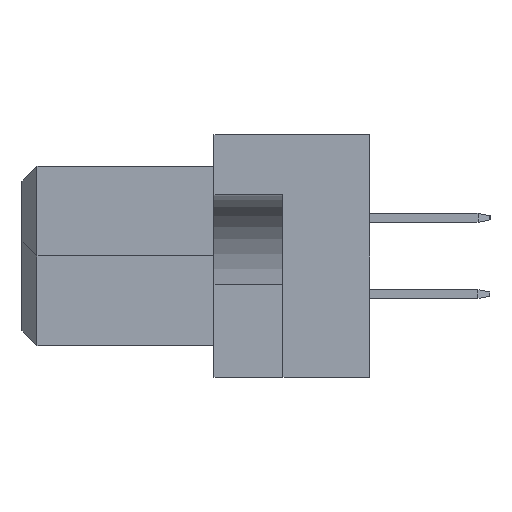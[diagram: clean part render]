
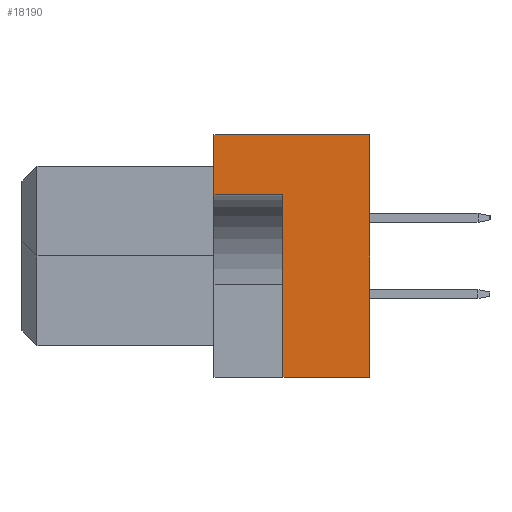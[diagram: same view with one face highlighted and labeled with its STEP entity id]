
A CAD part, left-side view. The second image highlights one B-rep face of the part: STEP entity #18190.
In plain terms, the highlighted planar face has unit normal (-1, 0, 0).
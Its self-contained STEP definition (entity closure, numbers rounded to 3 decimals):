
#1 = DIRECTION ( 'NONE',  ( 0., -1., 0. ) ) ;
#298 = ORIENTED_EDGE ( 'NONE', *, *, #13408, .F. ) ;
#1016 = DIRECTION ( 'NONE',  ( 0., 0., 1. ) ) ;
#1240 = EDGE_CURVE ( 'NONE', #6533, #2608, #6975, .T. ) ;
#2170 = VECTOR ( 'NONE', #9838, 1000. ) ;
#2217 = EDGE_CURVE ( 'NONE', #17133, #14557, #4733, .T. ) ;
#2578 = ORIENTED_EDGE ( 'NONE', *, *, #9832, .F. ) ;
#2608 = VERTEX_POINT ( 'NONE', #17832 ) ;
#3569 = VERTEX_POINT ( 'NONE', #16800 ) ;
#3932 = CARTESIAN_POINT ( 'NONE',  ( -35.12, 5.2, 4.05 ) ) ;
#4733 = LINE ( 'NONE', #7299, #18823 ) ;
#5071 = LINE ( 'NONE', #18130, #11200 ) ;
#5122 = LINE ( 'NONE', #11307, #8209 ) ;
#5419 = VECTOR ( 'NONE', #10106, 1000. ) ;
#5807 = ORIENTED_EDGE ( 'NONE', *, *, #1240, .F. ) ;
#5900 = FACE_OUTER_BOUND ( 'NONE', #15479, .T. ) ;
#6423 = CARTESIAN_POINT ( 'NONE',  ( -35.12, 5.2, 4.05 ) ) ;
#6533 = VERTEX_POINT ( 'NONE', #6423 ) ;
#6975 = LINE ( 'NONE', #10017, #15458 ) ;
#7299 = CARTESIAN_POINT ( 'NONE',  ( -35.12, 5.2, -4.05 ) ) ;
#8209 = VECTOR ( 'NONE', #1016, 1000. ) ;
#8859 = CARTESIAN_POINT ( 'NONE',  ( -35.12, 5.2, 4.05 ) ) ;
#8999 = AXIS2_PLACEMENT_3D ( 'NONE', #8859, #16206, #16406 ) ;
#9381 = VERTEX_POINT ( 'NONE', #15593 ) ;
#9832 = EDGE_CURVE ( 'NONE', #17133, #3569, #9928, .T. ) ;
#9838 = DIRECTION ( 'NONE',  ( 0., 0., 1. ) ) ;
#9928 = LINE ( 'NONE', #14217, #2170 ) ;
#10017 = CARTESIAN_POINT ( 'NONE',  ( -35.12, 5.2, 4.05 ) ) ;
#10106 = DIRECTION ( 'NONE',  ( 0., 0., 1. ) ) ;
#10443 = CARTESIAN_POINT ( 'NONE',  ( -35.12, 0., -4.05 ) ) ;
#11200 = VECTOR ( 'NONE', #16701, 1000. ) ;
#11307 = CARTESIAN_POINT ( 'NONE',  ( -35.12, 0., 4.05 ) ) ;
#11652 = ORIENTED_EDGE ( 'NONE', *, *, #13481, .F. ) ;
#12466 = CARTESIAN_POINT ( 'NONE',  ( -35.12, 2.9, -4.05 ) ) ;
#13055 = ORIENTED_EDGE ( 'NONE', *, *, #2217, .T. ) ;
#13408 = EDGE_CURVE ( 'NONE', #3569, #9381, #5071, .T. ) ;
#13481 = EDGE_CURVE ( 'NONE', #9381, #6533, #15637, .T. ) ;
#14217 = CARTESIAN_POINT ( 'NONE',  ( -35.12, 2.9, 2.05 ) ) ;
#14557 = VERTEX_POINT ( 'NONE', #10443 ) ;
#15458 = VECTOR ( 'NONE', #1, 1000. ) ;
#15479 = EDGE_LOOP ( 'NONE', ( #11652, #298, #2578, #13055, #18679, #5807 ) ) ;
#15593 = CARTESIAN_POINT ( 'NONE',  ( -35.12, 5.2, 2.05 ) ) ;
#15637 = LINE ( 'NONE', #3932, #5419 ) ;
#16206 = DIRECTION ( 'NONE',  ( 1., 0., 0. ) ) ;
#16357 = DIRECTION ( 'NONE',  ( 0., -1., 0. ) ) ;
#16406 = DIRECTION ( 'NONE',  ( 0., 0., -1. ) ) ;
#16701 = DIRECTION ( 'NONE',  ( 0., 1., 0. ) ) ;
#16800 = CARTESIAN_POINT ( 'NONE',  ( -35.12, 2.9, 2.05 ) ) ;
#17079 = EDGE_CURVE ( 'NONE', #14557, #2608, #5122, .T. ) ;
#17133 = VERTEX_POINT ( 'NONE', #12466 ) ;
#17532 = PLANE ( 'NONE',  #8999 ) ;
#17832 = CARTESIAN_POINT ( 'NONE',  ( -35.12, 0., 4.05 ) ) ;
#18130 = CARTESIAN_POINT ( 'NONE',  ( -35.12, 2.9, 2.05 ) ) ;
#18190 = ADVANCED_FACE ( 'NONE', ( #5900 ), #17532, .F. ) ;
#18679 = ORIENTED_EDGE ( 'NONE', *, *, #17079, .T. ) ;
#18823 = VECTOR ( 'NONE', #16357, 1000. ) ;
